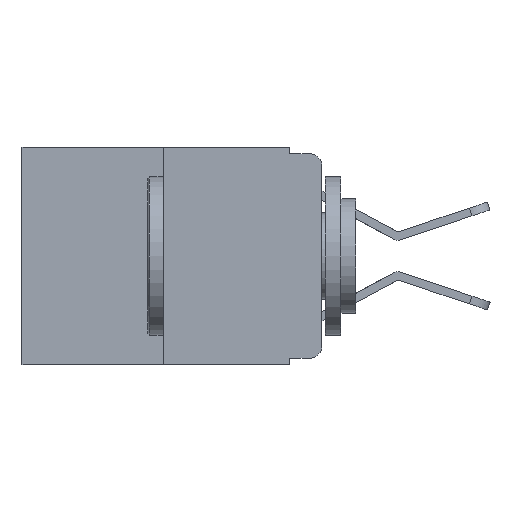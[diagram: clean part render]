
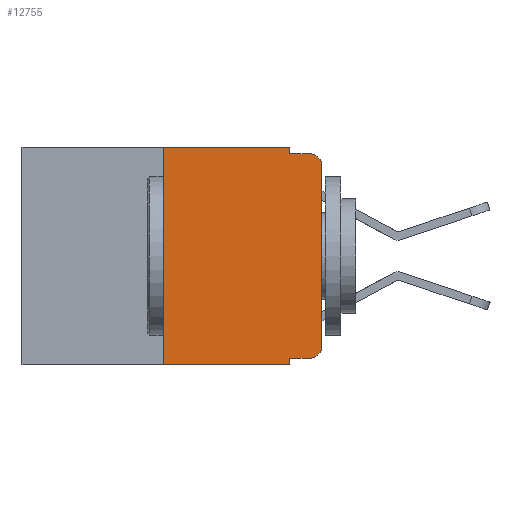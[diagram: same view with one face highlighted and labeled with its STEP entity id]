
A CAD part, left-side view. The second image highlights one B-rep face of the part: STEP entity #12755.
In plain terms, the highlighted planar face has unit normal (-1, 0, 0).
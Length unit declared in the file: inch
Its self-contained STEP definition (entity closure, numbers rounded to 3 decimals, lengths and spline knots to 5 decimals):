
#13 = CARTESIAN_POINT ( 'NONE',  ( 0., 0.051, 0. ) ) ;
#124 = CARTESIAN_POINT ( 'NONE',  ( 0., 0.051, 0. ) ) ;
#408 = AXIS2_PLACEMENT_3D ( 'NONE', #500, #10612, #11633 ) ;
#500 = CARTESIAN_POINT ( 'NONE',  ( 0., 0.02, -0.313 ) ) ;
#591 = ORIENTED_EDGE ( 'NONE', *, *, #5771, .F. ) ;
#1249 = ORIENTED_EDGE ( 'NONE', *, *, #6436, .T. ) ;
#1622 = DIRECTION ( 'NONE',  ( 0., -1., 0. ) ) ;
#1685 = LINE ( 'NONE', #3362, #8721 ) ;
#2102 = EDGE_CURVE ( 'NONE', #7264, #11305, #7831, .T. ) ;
#2718 = VECTOR ( 'NONE', #8143, 39.37008 ) ;
#2797 = ORIENTED_EDGE ( 'NONE', *, *, #9064, .T. ) ;
#2923 = ORIENTED_EDGE ( 'NONE', *, *, #2102, .F. ) ;
#2988 = ORIENTED_EDGE ( 'NONE', *, *, #4956, .T. ) ;
#3090 = CARTESIAN_POINT ( 'NONE',  ( 0., 0.473, 0. ) ) ;
#3113 = DIRECTION ( 'NONE',  ( 0., 0., -1. ) ) ;
#3362 = CARTESIAN_POINT ( 'NONE',  ( 0., 0.051, -0.333 ) ) ;
#3379 = EDGE_CURVE ( 'NONE', #9965, #12759, #7622, .T. ) ;
#3554 = EDGE_CURVE ( 'NONE', #11192, #11237, #1685, .T. ) ;
#3600 = FACE_OUTER_BOUND ( 'NONE', #4533, .T. ) ;
#3621 = CARTESIAN_POINT ( 'NONE',  ( 0., 0.25, 0. ) ) ;
#3890 = CARTESIAN_POINT ( 'NONE',  ( 0., 0.25, 0. ) ) ;
#3958 = CARTESIAN_POINT ( 'NONE',  ( 0., 0., -0.313 ) ) ;
#4265 = VECTOR ( 'NONE', #12920, 39.37008 ) ;
#4533 = EDGE_LOOP ( 'NONE', ( #2988, #2797, #2923, #591, #9147, #5025, #1249, #8421, #6718, #7738 ) ) ;
#4702 = LINE ( 'NONE', #7428, #8469 ) ;
#4956 = EDGE_CURVE ( 'NONE', #11598, #9994, #11326, .T. ) ;
#5025 = ORIENTED_EDGE ( 'NONE', *, *, #3379, .F. ) ;
#5063 = AXIS2_PLACEMENT_3D ( 'NONE', #5222, #6238, #3113 ) ;
#5222 = CARTESIAN_POINT ( 'NONE',  ( 0., 0.02, -0.03 ) ) ;
#5259 = CARTESIAN_POINT ( 'NONE',  ( 0., 0.02, -0.333 ) ) ;
#5492 = DIRECTION ( 'NONE',  ( 0., 0., -1. ) ) ;
#5582 = CARTESIAN_POINT ( 'NONE',  ( 0., 0.473, 0. ) ) ;
#5771 = EDGE_CURVE ( 'NONE', #6810, #7264, #8033, .T. ) ;
#5826 = EDGE_CURVE ( 'NONE', #12759, #6810, #7541, .T. ) ;
#5938 = DIRECTION ( 'NONE',  ( 0., 0., 1. ) ) ;
#6087 = CARTESIAN_POINT ( 'NONE',  ( 0., 0.051, 0. ) ) ;
#6238 = DIRECTION ( 'NONE',  ( -1., 0., 0. ) ) ;
#6254 = VECTOR ( 'NONE', #1622, 39.37008 ) ;
#6277 = CARTESIAN_POINT ( 'NONE',  ( 0., 0.051, -0.333 ) ) ;
#6436 = EDGE_CURVE ( 'NONE', #9965, #8718, #4702, .T. ) ;
#6718 = ORIENTED_EDGE ( 'NONE', *, *, #3554, .T. ) ;
#6783 = AXIS2_PLACEMENT_3D ( 'NONE', #5582, #10560, #5492 ) ;
#6810 = VERTEX_POINT ( 'NONE', #6087 ) ;
#7264 = VERTEX_POINT ( 'NONE', #12232 ) ;
#7428 = CARTESIAN_POINT ( 'NONE',  ( 0., 0.473, -0.343 ) ) ;
#7541 = LINE ( 'NONE', #3090, #11285 ) ;
#7622 = LINE ( 'NONE', #3890, #10758 ) ;
#7738 = ORIENTED_EDGE ( 'NONE', *, *, #8573, .T. ) ;
#7831 = LINE ( 'NONE', #9774, #6254 ) ;
#7949 = CARTESIAN_POINT ( 'NONE',  ( 0., 0., 0. ) ) ;
#8033 = LINE ( 'NONE', #124, #2718 ) ;
#8143 = DIRECTION ( 'NONE',  ( 0., 0., -1. ) ) ;
#8421 = ORIENTED_EDGE ( 'NONE', *, *, #11075, .F. ) ;
#8458 = DIRECTION ( 'NONE',  ( 0., -1., 0. ) ) ;
#8469 = VECTOR ( 'NONE', #8458, 39.37008 ) ;
#8573 = EDGE_CURVE ( 'NONE', #11237, #11598, #10748, .T. ) ;
#8718 = VERTEX_POINT ( 'NONE', #9649 ) ;
#8721 = VECTOR ( 'NONE', #10293, 39.37008 ) ;
#9064 = EDGE_CURVE ( 'NONE', #9994, #11305, #10104, .T. ) ;
#9147 = ORIENTED_EDGE ( 'NONE', *, *, #5826, .F. ) ;
#9584 = CARTESIAN_POINT ( 'NONE',  ( 0., 0.25, -0.343 ) ) ;
#9625 = CARTESIAN_POINT ( 'NONE',  ( 0., 0., -0.03 ) ) ;
#9640 = PLANE ( 'NONE',  #6783 ) ;
#9649 = CARTESIAN_POINT ( 'NONE',  ( 0., 0.051, -0.343 ) ) ;
#9774 = CARTESIAN_POINT ( 'NONE',  ( 0., 0.051, -0.01 ) ) ;
#9965 = VERTEX_POINT ( 'NONE', #9584 ) ;
#9994 = VERTEX_POINT ( 'NONE', #9625 ) ;
#10104 = CIRCLE ( 'NONE', #5063, 0.02 ) ;
#10221 = DIRECTION ( 'NONE',  ( 0., -1., 0. ) ) ;
#10293 = DIRECTION ( 'NONE',  ( 0., -1., 0. ) ) ;
#10560 = DIRECTION ( 'NONE',  ( 1., 0., 0. ) ) ;
#10612 = DIRECTION ( 'NONE',  ( -1., 0., 0. ) ) ;
#10748 = CIRCLE ( 'NONE', #408, 0.02 ) ;
#10758 = VECTOR ( 'NONE', #10962, 39.37008 ) ;
#10838 = LINE ( 'NONE', #13, #4265 ) ;
#10962 = DIRECTION ( 'NONE',  ( 0., 0., 1. ) ) ;
#11075 = EDGE_CURVE ( 'NONE', #11192, #8718, #10838, .T. ) ;
#11192 = VERTEX_POINT ( 'NONE', #6277 ) ;
#11237 = VERTEX_POINT ( 'NONE', #5259 ) ;
#11285 = VECTOR ( 'NONE', #10221, 39.37008 ) ;
#11305 = VERTEX_POINT ( 'NONE', #11472 ) ;
#11326 = LINE ( 'NONE', #7949, #12740 ) ;
#11472 = CARTESIAN_POINT ( 'NONE',  ( 0., 0.02, -0.01 ) ) ;
#11598 = VERTEX_POINT ( 'NONE', #3958 ) ;
#11633 = DIRECTION ( 'NONE',  ( 0., 0., -1. ) ) ;
#12232 = CARTESIAN_POINT ( 'NONE',  ( 0., 0.051, -0.01 ) ) ;
#12740 = VECTOR ( 'NONE', #5938, 39.37008 ) ;
#12755 = ADVANCED_FACE ( 'NONE', ( #3600 ), #9640, .F. ) ;
#12759 = VERTEX_POINT ( 'NONE', #3621 ) ;
#12920 = DIRECTION ( 'NONE',  ( 0., 0., -1. ) ) ;
